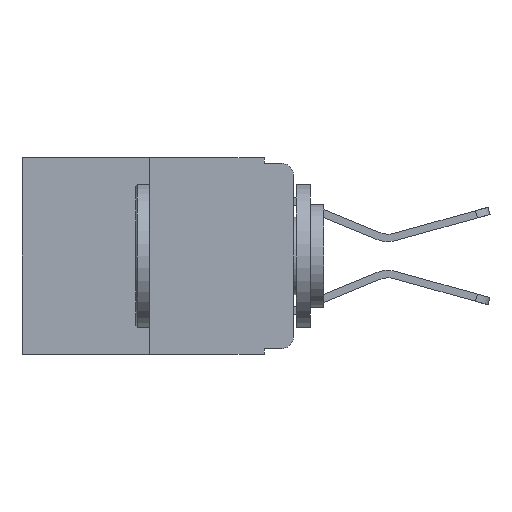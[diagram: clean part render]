
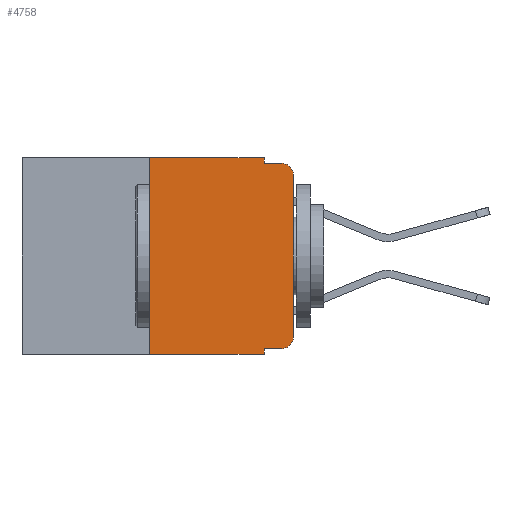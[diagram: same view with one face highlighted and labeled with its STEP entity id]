
A CAD part, left-side view. The second image highlights one B-rep face of the part: STEP entity #4758.
In plain terms, the highlighted planar face has unit normal (-1, 0, 0).
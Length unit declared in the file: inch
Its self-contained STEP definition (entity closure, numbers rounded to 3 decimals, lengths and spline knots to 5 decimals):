
#2 = CARTESIAN_POINT ( 'NONE',  ( 0., 0.25, -0.343 ) ) ;
#78 = AXIS2_PLACEMENT_3D ( 'NONE', #7789, #2072, #8689 ) ;
#333 = DIRECTION ( 'NONE',  ( 0., 0., -1. ) ) ;
#357 = EDGE_CURVE ( 'NONE', #4077, #1941, #3420, .T. ) ;
#412 = DIRECTION ( 'NONE',  ( -1., 0., 0. ) ) ;
#678 = EDGE_CURVE ( 'NONE', #1885, #1881, #2663, .T. ) ;
#935 = CARTESIAN_POINT ( 'NONE',  ( 0., 0.473, 0. ) ) ;
#958 = CARTESIAN_POINT ( 'NONE',  ( 0., 0.051, -0.01 ) ) ;
#969 = DIRECTION ( 'NONE',  ( 0., 0., -1. ) ) ;
#1118 = EDGE_CURVE ( 'NONE', #1885, #8504, #5219, .T. ) ;
#1392 = CARTESIAN_POINT ( 'NONE',  ( 0., 0.02, -0.333 ) ) ;
#1483 = CARTESIAN_POINT ( 'NONE',  ( 0., 0.25, 0. ) ) ;
#1519 = CARTESIAN_POINT ( 'NONE',  ( 0., 0.02, -0.01 ) ) ;
#1525 = DIRECTION ( 'NONE',  ( 0., -1., 0. ) ) ;
#1881 = VERTEX_POINT ( 'NONE', #1392 ) ;
#1885 = VERTEX_POINT ( 'NONE', #6521 ) ;
#1941 = VERTEX_POINT ( 'NONE', #11050 ) ;
#2010 = LINE ( 'NONE', #5403, #11508 ) ;
#2072 = DIRECTION ( 'NONE',  ( -1., 0., 0. ) ) ;
#2154 = CIRCLE ( 'NONE', #11358, 0.02 ) ;
#2432 = EDGE_CURVE ( 'NONE', #4264, #3561, #9855, .T. ) ;
#2564 = CARTESIAN_POINT ( 'NONE',  ( 0., 0.051, -0.01 ) ) ;
#2595 = CARTESIAN_POINT ( 'NONE',  ( 0., 0.25, 0. ) ) ;
#2663 = LINE ( 'NONE', #5484, #7723 ) ;
#2695 = CARTESIAN_POINT ( 'NONE',  ( 0., 0.473, 0. ) ) ;
#2918 = ORIENTED_EDGE ( 'NONE', *, *, #10336, .F. ) ;
#3095 = LINE ( 'NONE', #2695, #9888 ) ;
#3221 = ORIENTED_EDGE ( 'NONE', *, *, #6942, .F. ) ;
#3412 = VERTEX_POINT ( 'NONE', #2595 ) ;
#3420 = LINE ( 'NONE', #10821, #6288 ) ;
#3561 = VERTEX_POINT ( 'NONE', #1519 ) ;
#3653 = DIRECTION ( 'NONE',  ( 0., -1., 0. ) ) ;
#3656 = VERTEX_POINT ( 'NONE', #4779 ) ;
#3676 = LINE ( 'NONE', #6186, #6541 ) ;
#4077 = VERTEX_POINT ( 'NONE', #5939 ) ;
#4264 = VERTEX_POINT ( 'NONE', #958 ) ;
#4421 = ORIENTED_EDGE ( 'NONE', *, *, #1118, .F. ) ;
#4574 = ORIENTED_EDGE ( 'NONE', *, *, #2432, .F. ) ;
#4718 = VECTOR ( 'NONE', #7767, 39.37008 ) ;
#4758 = ADVANCED_FACE ( 'NONE', ( #6899 ), #5821, .F. ) ;
#4779 = CARTESIAN_POINT ( 'NONE',  ( 0., 0.051, 0. ) ) ;
#5219 = LINE ( 'NONE', #10083, #9765 ) ;
#5403 = CARTESIAN_POINT ( 'NONE',  ( 0., 0.473, -0.343 ) ) ;
#5484 = CARTESIAN_POINT ( 'NONE',  ( 0., 0.051, -0.333 ) ) ;
#5821 = PLANE ( 'NONE',  #8627 ) ;
#5939 = CARTESIAN_POINT ( 'NONE',  ( 0., 0., -0.313 ) ) ;
#6186 = CARTESIAN_POINT ( 'NONE',  ( 0., 0.051, 0. ) ) ;
#6253 = CARTESIAN_POINT ( 'NONE',  ( 0., 0.02, -0.03 ) ) ;
#6288 = VECTOR ( 'NONE', #10832, 39.37008 ) ;
#6513 = EDGE_LOOP ( 'NONE', ( #10532, #9057, #4574, #9727, #2918, #3221, #10820, #4421, #9604, #9872 ) ) ;
#6521 = CARTESIAN_POINT ( 'NONE',  ( 0., 0.051, -0.333 ) ) ;
#6541 = VECTOR ( 'NONE', #333, 39.37008 ) ;
#6785 = DIRECTION ( 'NONE',  ( 0., 0., -1. ) ) ;
#6899 = FACE_OUTER_BOUND ( 'NONE', #6513, .T. ) ;
#6942 = EDGE_CURVE ( 'NONE', #8207, #3412, #9748, .T. ) ;
#6954 = EDGE_CURVE ( 'NONE', #8207, #8504, #2010, .T. ) ;
#7127 = VECTOR ( 'NONE', #9054, 39.37008 ) ;
#7155 = CIRCLE ( 'NONE', #78, 0.02 ) ;
#7184 = DIRECTION ( 'NONE',  ( 0., 0., -1. ) ) ;
#7723 = VECTOR ( 'NONE', #8898, 39.37008 ) ;
#7767 = DIRECTION ( 'NONE',  ( 0., -1., 0. ) ) ;
#7789 = CARTESIAN_POINT ( 'NONE',  ( 0., 0.02, -0.313 ) ) ;
#8207 = VERTEX_POINT ( 'NONE', #2 ) ;
#8504 = VERTEX_POINT ( 'NONE', #10773 ) ;
#8627 = AXIS2_PLACEMENT_3D ( 'NONE', #935, #12054, #6785 ) ;
#8689 = DIRECTION ( 'NONE',  ( 0., 0., -1. ) ) ;
#8898 = DIRECTION ( 'NONE',  ( 0., -1., 0. ) ) ;
#9054 = DIRECTION ( 'NONE',  ( 0., 0., 1. ) ) ;
#9057 = ORIENTED_EDGE ( 'NONE', *, *, #11212, .T. ) ;
#9370 = EDGE_CURVE ( 'NONE', #1881, #4077, #7155, .T. ) ;
#9604 = ORIENTED_EDGE ( 'NONE', *, *, #678, .T. ) ;
#9727 = ORIENTED_EDGE ( 'NONE', *, *, #10674, .F. ) ;
#9748 = LINE ( 'NONE', #1483, #7127 ) ;
#9765 = VECTOR ( 'NONE', #969, 39.37008 ) ;
#9855 = LINE ( 'NONE', #2564, #4718 ) ;
#9872 = ORIENTED_EDGE ( 'NONE', *, *, #9370, .T. ) ;
#9888 = VECTOR ( 'NONE', #3653, 39.37008 ) ;
#10083 = CARTESIAN_POINT ( 'NONE',  ( 0., 0.051, 0. ) ) ;
#10336 = EDGE_CURVE ( 'NONE', #3412, #3656, #3095, .T. ) ;
#10532 = ORIENTED_EDGE ( 'NONE', *, *, #357, .T. ) ;
#10674 = EDGE_CURVE ( 'NONE', #3656, #4264, #3676, .T. ) ;
#10773 = CARTESIAN_POINT ( 'NONE',  ( 0., 0.051, -0.343 ) ) ;
#10820 = ORIENTED_EDGE ( 'NONE', *, *, #6954, .T. ) ;
#10821 = CARTESIAN_POINT ( 'NONE',  ( 0., 0., 0. ) ) ;
#10832 = DIRECTION ( 'NONE',  ( 0., 0., 1. ) ) ;
#11050 = CARTESIAN_POINT ( 'NONE',  ( 0., 0., -0.03 ) ) ;
#11212 = EDGE_CURVE ( 'NONE', #1941, #3561, #2154, .T. ) ;
#11358 = AXIS2_PLACEMENT_3D ( 'NONE', #6253, #412, #7184 ) ;
#11508 = VECTOR ( 'NONE', #1525, 39.37008 ) ;
#12054 = DIRECTION ( 'NONE',  ( 1., 0., 0. ) ) ;
